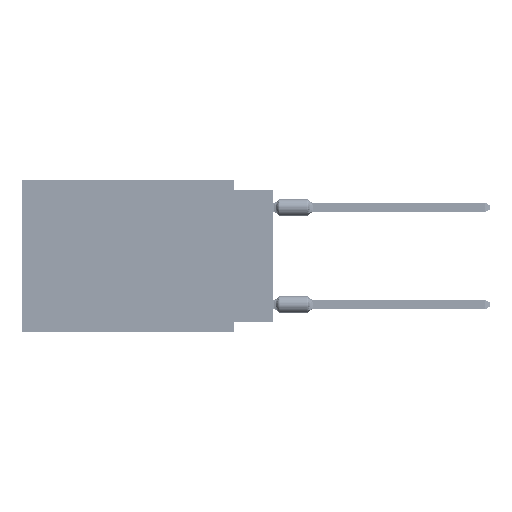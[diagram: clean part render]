
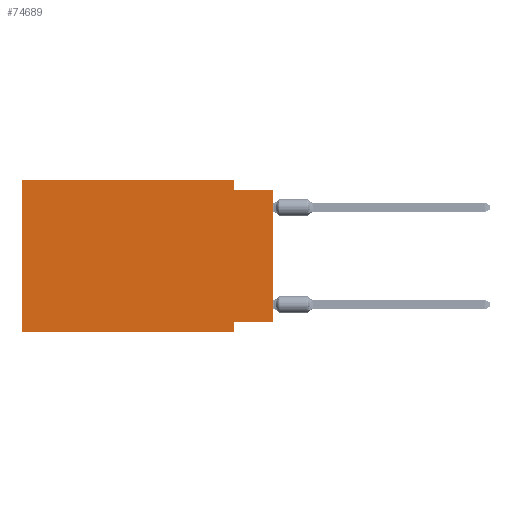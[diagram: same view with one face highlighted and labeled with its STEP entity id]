
A CAD part, left-side view. The second image highlights one B-rep face of the part: STEP entity #74689.
In plain terms, the highlighted planar face has unit normal (-1, 0, 0).
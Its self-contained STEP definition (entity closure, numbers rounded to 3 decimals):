
#732 = CARTESIAN_POINT ( 'NONE',  ( 0., 0., -9.271 ) ) ;
#3522 = CARTESIAN_POINT ( 'NONE',  ( 0., 0., -9.271 ) ) ;
#4011 = CARTESIAN_POINT ( 'NONE',  ( 0., 2.54, -9.271 ) ) ;
#4774 = EDGE_CURVE ( 'NONE', #73254, #15739, #50403, .T. ) ;
#5098 = ORIENTED_EDGE ( 'NONE', *, *, #74209, .F. ) ;
#5837 = CARTESIAN_POINT ( 'NONE',  ( 0., 0., -0.635 ) ) ;
#10176 = ORIENTED_EDGE ( 'NONE', *, *, #4774, .F. ) ;
#11765 = LINE ( 'NONE', #18255, #51596 ) ;
#12723 = CARTESIAN_POINT ( 'NONE',  ( 0., 2.54, -0.635 ) ) ;
#12898 = PLANE ( 'NONE',  #73313 ) ;
#13135 = VECTOR ( 'NONE', #73900, 1000. ) ;
#13145 = VECTOR ( 'NONE', #13336, 1000. ) ;
#13336 = DIRECTION ( 'NONE',  ( 0., 1., 0. ) ) ;
#13439 = CARTESIAN_POINT ( 'NONE',  ( 0., 2.54, 0. ) ) ;
#15040 = EDGE_CURVE ( 'NONE', #17002, #51336, #43501, .T. ) ;
#15739 = VERTEX_POINT ( 'NONE', #12723 ) ;
#15855 = CARTESIAN_POINT ( 'NONE',  ( 0., 16.383, 0. ) ) ;
#16073 = CARTESIAN_POINT ( 'NONE',  ( 0., 2.54, 0. ) ) ;
#17002 = VERTEX_POINT ( 'NONE', #3522 ) ;
#18255 = CARTESIAN_POINT ( 'NONE',  ( 0., 2.54, -9.906 ) ) ;
#19081 = LINE ( 'NONE', #49955, #64248 ) ;
#19509 = CARTESIAN_POINT ( 'NONE',  ( 0., 0., 0. ) ) ;
#20124 = CARTESIAN_POINT ( 'NONE',  ( 0., 16.383, -9.906 ) ) ;
#20960 = DIRECTION ( 'NONE',  ( 0., -1., 0. ) ) ;
#22184 = EDGE_CURVE ( 'NONE', #34456, #47416, #76536, .T. ) ;
#24297 = DIRECTION ( 'NONE',  ( 0., 0., -1. ) ) ;
#24848 = ORIENTED_EDGE ( 'NONE', *, *, #15040, .T. ) ;
#25156 = VECTOR ( 'NONE', #30629, 1000. ) ;
#30629 = DIRECTION ( 'NONE',  ( 0., -1., 0. ) ) ;
#32346 = CARTESIAN_POINT ( 'NONE',  ( 0., 16.383, -9.906 ) ) ;
#33155 = VECTOR ( 'NONE', #50786, 1000. ) ;
#34240 = ORIENTED_EDGE ( 'NONE', *, *, #69423, .F. ) ;
#34456 = VERTEX_POINT ( 'NONE', #20124 ) ;
#38222 = DIRECTION ( 'NONE',  ( 0., 0., -1. ) ) ;
#40272 = ORIENTED_EDGE ( 'NONE', *, *, #72403, .F. ) ;
#41270 = EDGE_CURVE ( 'NONE', #56932, #47416, #11765, .T. ) ;
#41315 = VECTOR ( 'NONE', #20960, 1000. ) ;
#42784 = ORIENTED_EDGE ( 'NONE', *, *, #22184, .T. ) ;
#43368 = DIRECTION ( 'NONE',  ( 1., 0., 0. ) ) ;
#43501 = LINE ( 'NONE', #19509, #33155 ) ;
#47416 = VERTEX_POINT ( 'NONE', #64672 ) ;
#47939 = VERTEX_POINT ( 'NONE', #15855 ) ;
#49197 = CARTESIAN_POINT ( 'NONE',  ( 0., 16.383, 0. ) ) ;
#49955 = CARTESIAN_POINT ( 'NONE',  ( 0., 16.383, 0. ) ) ;
#50403 = LINE ( 'NONE', #13439, #61420 ) ;
#50786 = DIRECTION ( 'NONE',  ( 0., 0., 1. ) ) ;
#51336 = VERTEX_POINT ( 'NONE', #62379 ) ;
#51596 = VECTOR ( 'NONE', #73043, 1000. ) ;
#53556 = ORIENTED_EDGE ( 'NONE', *, *, #41270, .F. ) ;
#55207 = EDGE_CURVE ( 'NONE', #34456, #47939, #65836, .T. ) ;
#56932 = VERTEX_POINT ( 'NONE', #4011 ) ;
#57139 = FACE_OUTER_BOUND ( 'NONE', #63681, .T. ) ;
#61420 = VECTOR ( 'NONE', #38222, 1000. ) ;
#61476 = LINE ( 'NONE', #5837, #25156 ) ;
#61736 = DIRECTION ( 'NONE',  ( 0., -1., 0. ) ) ;
#62379 = CARTESIAN_POINT ( 'NONE',  ( 0., 0., -0.635 ) ) ;
#63681 = EDGE_LOOP ( 'NONE', ( #24848, #40272, #10176, #5098, #68654, #42784, #53556, #34240 ) ) ;
#64248 = VECTOR ( 'NONE', #61736, 1000. ) ;
#64672 = CARTESIAN_POINT ( 'NONE',  ( 0., 2.54, -9.906 ) ) ;
#65836 = LINE ( 'NONE', #49197, #13135 ) ;
#68654 = ORIENTED_EDGE ( 'NONE', *, *, #55207, .F. ) ;
#69284 = CARTESIAN_POINT ( 'NONE',  ( 0., 16.383, 0. ) ) ;
#69423 = EDGE_CURVE ( 'NONE', #17002, #56932, #75013, .T. ) ;
#72403 = EDGE_CURVE ( 'NONE', #15739, #51336, #61476, .T. ) ;
#73043 = DIRECTION ( 'NONE',  ( 0., 0., -1. ) ) ;
#73254 = VERTEX_POINT ( 'NONE', #16073 ) ;
#73313 = AXIS2_PLACEMENT_3D ( 'NONE', #69284, #43368, #24297 ) ;
#73900 = DIRECTION ( 'NONE',  ( 0., 0., 1. ) ) ;
#74209 = EDGE_CURVE ( 'NONE', #47939, #73254, #19081, .T. ) ;
#74689 = ADVANCED_FACE ( 'NONE', ( #57139 ), #12898, .F. ) ;
#75013 = LINE ( 'NONE', #732, #13145 ) ;
#76536 = LINE ( 'NONE', #32346, #41315 ) ;
